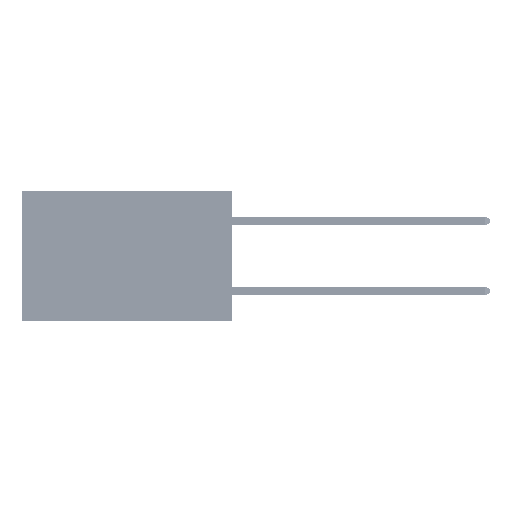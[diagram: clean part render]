
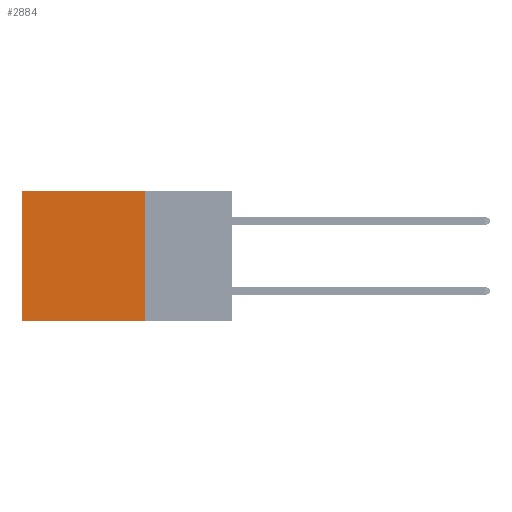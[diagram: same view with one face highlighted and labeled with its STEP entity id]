
A CAD part, left-side view. The second image highlights one B-rep face of the part: STEP entity #2884.
In plain terms, the highlighted planar face has unit normal (-1, 0, 0).
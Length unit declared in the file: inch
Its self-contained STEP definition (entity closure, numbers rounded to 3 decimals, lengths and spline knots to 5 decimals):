
#19 = CARTESIAN_POINT ( 'NONE',  ( 0.2875, 0.25, 0. ) ) ;
#797 = VECTOR ( 'NONE', #27326, 39.37008 ) ;
#916 = VERTEX_POINT ( 'NONE', #19632 ) ;
#1981 = LINE ( 'NONE', #42525, #3930 ) ;
#2710 = EDGE_LOOP ( 'NONE', ( #44118, #12529, #18178, #32406 ) ) ;
#2884 = ADVANCED_FACE ( 'NONE', ( #13622 ), #3761, .F. ) ;
#3761 = PLANE ( 'NONE',  #22904 ) ;
#3851 = DIRECTION ( 'NONE',  ( 0., 0., -1. ) ) ;
#3930 = VECTOR ( 'NONE', #32956, 39.37008 ) ;
#5210 = CARTESIAN_POINT ( 'NONE',  ( 0.2875, 0.6, 0. ) ) ;
#5833 = EDGE_CURVE ( 'NONE', #20037, #8859, #1981, .T. ) ;
#8288 = CARTESIAN_POINT ( 'NONE',  ( 0.2875, 0.25, 0. ) ) ;
#8859 = VERTEX_POINT ( 'NONE', #18133 ) ;
#11143 = EDGE_CURVE ( 'NONE', #41998, #916, #33679, .T. ) ;
#12529 = ORIENTED_EDGE ( 'NONE', *, *, #5833, .F. ) ;
#13622 = FACE_OUTER_BOUND ( 'NONE', #2710, .T. ) ;
#18133 = CARTESIAN_POINT ( 'NONE',  ( 0.2875, 0.6, -0.37 ) ) ;
#18178 = ORIENTED_EDGE ( 'NONE', *, *, #37925, .F. ) ;
#18570 = LINE ( 'NONE', #40072, #30630 ) ;
#19632 = CARTESIAN_POINT ( 'NONE',  ( 0.2875, 0.6, 0. ) ) ;
#20037 = VERTEX_POINT ( 'NONE', #23004 ) ;
#22904 = AXIS2_PLACEMENT_3D ( 'NONE', #19, #36091, #48460 ) ;
#23004 = CARTESIAN_POINT ( 'NONE',  ( 0.2875, 0.25, -0.37 ) ) ;
#23269 = CARTESIAN_POINT ( 'NONE',  ( 0.2875, 0.25, 0. ) ) ;
#27326 = DIRECTION ( 'NONE',  ( 0., 1., 0. ) ) ;
#30630 = VECTOR ( 'NONE', #3851, 39.37008 ) ;
#32406 = ORIENTED_EDGE ( 'NONE', *, *, #11143, .T. ) ;
#32956 = DIRECTION ( 'NONE',  ( 0., 1., 0. ) ) ;
#33679 = LINE ( 'NONE', #23269, #797 ) ;
#36091 = DIRECTION ( 'NONE',  ( 1., 0., 0. ) ) ;
#37524 = DIRECTION ( 'NONE',  ( 0., 0., -1. ) ) ;
#37845 = LINE ( 'NONE', #5210, #51768 ) ;
#37925 = EDGE_CURVE ( 'NONE', #41998, #20037, #18570, .T. ) ;
#40072 = CARTESIAN_POINT ( 'NONE',  ( 0.2875, 0.25, 0. ) ) ;
#41998 = VERTEX_POINT ( 'NONE', #8288 ) ;
#42525 = CARTESIAN_POINT ( 'NONE',  ( 0.2875, 0.25, -0.37 ) ) ;
#44118 = ORIENTED_EDGE ( 'NONE', *, *, #52056, .T. ) ;
#48460 = DIRECTION ( 'NONE',  ( 0., 0., -1. ) ) ;
#51768 = VECTOR ( 'NONE', #37524, 39.37008 ) ;
#52056 = EDGE_CURVE ( 'NONE', #916, #8859, #37845, .T. ) ;
